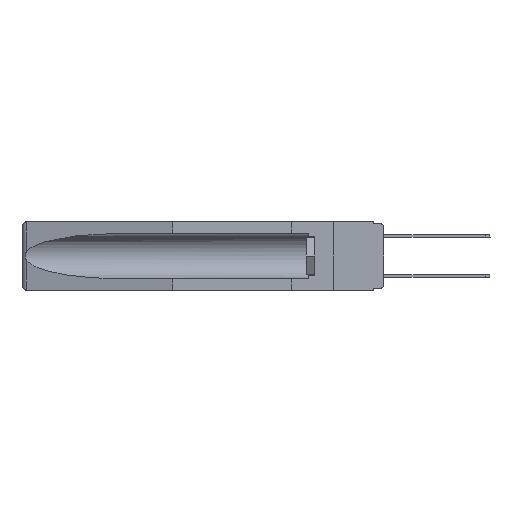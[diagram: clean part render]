
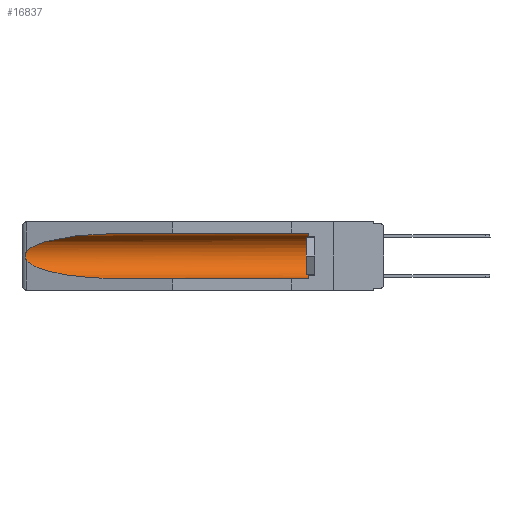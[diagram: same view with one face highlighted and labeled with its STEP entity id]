
A CAD part, left-side view. The second image highlights one B-rep face of the part: STEP entity #16837.
In plain terms, the highlighted cylindrical face has radius 2.857 mm (diameter 5.715 mm), a partial arc.
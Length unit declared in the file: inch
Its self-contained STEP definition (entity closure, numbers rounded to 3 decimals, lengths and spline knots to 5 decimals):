
#501 = EDGE_LOOP ( 'NONE', ( #6492, #14559, #10960, #18787, #1351, #21152 ) ) ;
#1101 = VERTEX_POINT ( 'NONE', #17793 ) ;
#1160 = CYLINDRICAL_SURFACE ( 'NONE', #17076, 0.1125 ) ;
#1351 = ORIENTED_EDGE ( 'NONE', *, *, #16211, .T. ) ;
#2239 = CARTESIAN_POINT ( 'NONE',  ( 0.25451, 1.48313, -0.09465 ) ) ;
#2744 = CARTESIAN_POINT ( 'NONE',  ( 0.155, 1.07973, -0.284 ) ) ;
#2842 = CARTESIAN_POINT ( 'NONE',  ( 0.155, 0.126, -0.059 ) ) ;
#2851 = EDGE_CURVE ( 'NONE', #21592, #7401, #5498, .T. ) ;
#3176 = CARTESIAN_POINT ( 'NONE',  ( 0.26655, 1.53094, -0.18657 ) ) ;
#3289 = CARTESIAN_POINT ( 'NONE',  ( 0.26537, 1.52718, -0.19328 ) ) ;
#3381 = CARTESIAN_POINT ( 'NONE',  ( 0.155, -0.30754, -0.1715 ) ) ;
#3398 = CARTESIAN_POINT ( 'NONE',  ( 0.26654, 1.53092, -0.15636 ) ) ;
#3540 = CARTESIAN_POINT ( 'NONE',  ( 0.26597, 1.52961, -0.15275 ) ) ;
#3647 = CARTESIAN_POINT ( 'NONE',  ( 0.26537, 1.52718, -0.14972 ) ) ;
#4511 = CARTESIAN_POINT ( 'NONE',  ( 0.155, 1.07973, -0.284 ) ) ;
#4593 = DIRECTION ( 'NONE',  ( 0., 1., 0. ) ) ;
#4697 = VERTEX_POINT ( 'NONE', #3647 ) ;
#4969 = DIRECTION ( 'NONE',  ( 0., 1., 0. ) ) ;
#5140 = B_SPLINE_CURVE_WITH_KNOTS ( 'NONE', 3,
 ( #6745, #3540, #3398, #10256, #11695, #8396, #13373, #3176, #9957, #6523 ),
 .UNSPECIFIED., .F., .F.,
 ( 4, 2, 2, 2, 4 ),
 ( 0., 0.00029, 0.00058, 0.00087, 0.00117 ),
 .UNSPECIFIED. ) ;
#5250 = EDGE_CURVE ( 'NONE', #4697, #18769, #5140, .T. ) ;
#5498 = LINE ( 'NONE', #21477, #15410 ) ;
#6492 = ORIENTED_EDGE ( 'NONE', *, *, #12501, .T. ) ;
#6523 = CARTESIAN_POINT ( 'NONE',  ( 0.26537, 1.52718, -0.19328 ) ) ;
#6689 = DIRECTION ( 'NONE',  ( 0., -1., 0. ) ) ;
#6745 = CARTESIAN_POINT ( 'NONE',  ( 0.26537, 1.52718, -0.14972 ) ) ;
#6755 = DIRECTION ( 'NONE',  ( 0., 0., 1. ) ) ;
#6762 = CARTESIAN_POINT ( 'NONE',  ( 0.155, 1.07973, -0.059 ) ) ;
#7401 = VERTEX_POINT ( 'NONE', #6762 ) ;
#8079 = EDGE_CURVE ( 'NONE', #1101, #14539, #11759, .T. ) ;
#8396 = CARTESIAN_POINT ( 'NONE',  ( 0.2675, 1.53308, -0.17534 ) ) ;
#8623 = CARTESIAN_POINT ( 'NONE',  ( 0.155, 0.126, -0.1715 ) ) ;
#8907 = FACE_OUTER_BOUND ( 'NONE', #501, .T. ) ;
#9799 = CARTESIAN_POINT ( 'NONE',  ( 0.26537, 1.52718, -0.19328 ) ) ;
#9957 = CARTESIAN_POINT ( 'NONE',  ( 0.26597, 1.5296, -0.19026 ) ) ;
#10256 = CARTESIAN_POINT ( 'NONE',  ( 0.2673, 1.5327, -0.16383 ) ) ;
#10960 = ORIENTED_EDGE ( 'NONE', *, *, #19823, .T. ) ;
#11311 = CARTESIAN_POINT ( 'NONE',  ( 0.25451, 1.48313, -0.24835 ) ) ;
#11695 = CARTESIAN_POINT ( 'NONE',  ( 0.2675, 1.53308, -0.16763 ) ) ;
#11759 = LINE ( 'NONE', #22048, #19291 ) ;
#12271 = CARTESIAN_POINT ( 'NONE',  ( 0.26537, 1.52718, -0.14972 ) ) ;
#12422 = CIRCLE ( 'NONE', #17494, 0.1125 ) ;
#12501 = EDGE_CURVE ( 'NONE', #7401, #4697, #15453, .T. ) ;
#13373 = CARTESIAN_POINT ( 'NONE',  ( 0.2673, 1.53269, -0.17917 ) ) ;
#14348 =( BOUNDED_CURVE ( )  B_SPLINE_CURVE ( 3, ( #9799, #11311, #14777, #4511 ),
 .UNSPECIFIED., .F., .F. ) 
 B_SPLINE_CURVE_WITH_KNOTS ( ( 4, 4 ),
 ( 0.1948, 1.5708 ),
 .UNSPECIFIED. ) 
 CURVE ( )  GEOMETRIC_REPRESENTATION_ITEM ( )  RATIONAL_B_SPLINE_CURVE ( ( 1., 0.848, 0.848, 1. ) ) 
 REPRESENTATION_ITEM ( '' )  );
#14539 = VERTEX_POINT ( 'NONE', #2744 ) ;
#14559 = ORIENTED_EDGE ( 'NONE', *, *, #5250, .T. ) ;
#14777 = CARTESIAN_POINT ( 'NONE',  ( 0.21114, 1.30732, -0.284 ) ) ;
#15410 = VECTOR ( 'NONE', #18171, 39.37008 ) ;
#15453 =( BOUNDED_CURVE ( )  B_SPLINE_CURVE ( 3, ( #17372, #20739, #2239, #12271 ),
 .UNSPECIFIED., .F., .F. ) 
 B_SPLINE_CURVE_WITH_KNOTS ( ( 4, 4 ),
 ( 4.71239, 6.08839 ),
 .UNSPECIFIED. ) 
 CURVE ( )  GEOMETRIC_REPRESENTATION_ITEM ( )  RATIONAL_B_SPLINE_CURVE ( ( 1., 0.848, 0.848, 1. ) ) 
 REPRESENTATION_ITEM ( '' )  );
#16211 = EDGE_CURVE ( 'NONE', #1101, #21592, #12422, .T. ) ;
#16837 = ADVANCED_FACE ( 'NONE', ( #8907 ), #1160, .F. ) ;
#17076 = AXIS2_PLACEMENT_3D ( 'NONE', #3381, #4969, #20323 ) ;
#17372 = CARTESIAN_POINT ( 'NONE',  ( 0.155, 1.07973, -0.059 ) ) ;
#17494 = AXIS2_PLACEMENT_3D ( 'NONE', #8623, #6689, #6755 ) ;
#17793 = CARTESIAN_POINT ( 'NONE',  ( 0.155, 0.126, -0.284 ) ) ;
#18171 = DIRECTION ( 'NONE',  ( 0., 1., 0. ) ) ;
#18769 = VERTEX_POINT ( 'NONE', #3289 ) ;
#18787 = ORIENTED_EDGE ( 'NONE', *, *, #8079, .F. ) ;
#19291 = VECTOR ( 'NONE', #4593, 39.37008 ) ;
#19823 = EDGE_CURVE ( 'NONE', #18769, #14539, #14348, .T. ) ;
#20323 = DIRECTION ( 'NONE',  ( 0., 0., 1. ) ) ;
#20739 = CARTESIAN_POINT ( 'NONE',  ( 0.21114, 1.30732, -0.059 ) ) ;
#21152 = ORIENTED_EDGE ( 'NONE', *, *, #2851, .T. ) ;
#21477 = CARTESIAN_POINT ( 'NONE',  ( 0.155, -0.30754, -0.059 ) ) ;
#21592 = VERTEX_POINT ( 'NONE', #2842 ) ;
#22048 = CARTESIAN_POINT ( 'NONE',  ( 0.155, -0.30754, -0.284 ) ) ;
